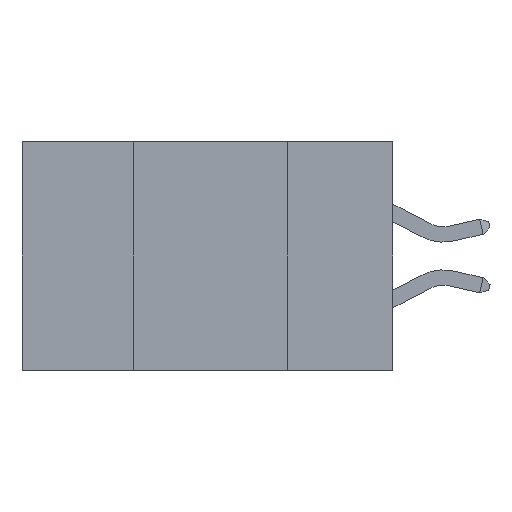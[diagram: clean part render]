
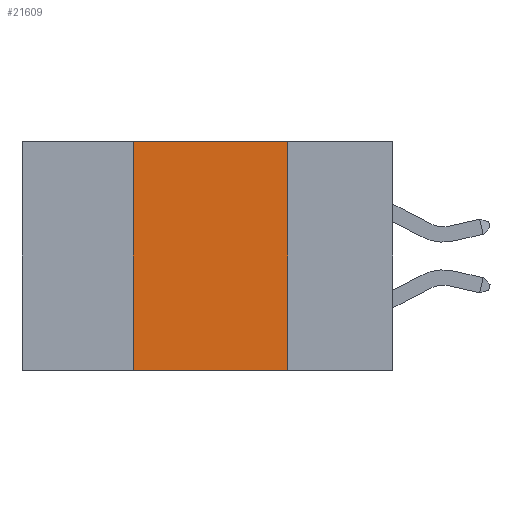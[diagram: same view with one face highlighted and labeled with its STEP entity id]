
A CAD part, left-side view. The second image highlights one B-rep face of the part: STEP entity #21609.
In plain terms, the highlighted planar face has unit normal (-1, 0, 0).
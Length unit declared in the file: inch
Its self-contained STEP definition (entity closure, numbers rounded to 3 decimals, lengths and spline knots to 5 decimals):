
#3584 = DIRECTION ( 'NONE',  ( 1., 0., 0. ) ) ;
#4067 = EDGE_CURVE ( 'NONE', #6951, #6620, #8706, .T. ) ;
#4097 = EDGE_CURVE ( 'NONE', #8169, #19442, #12816, .T. ) ;
#4108 = EDGE_CURVE ( 'NONE', #8169, #6620, #7633, .T. ) ;
#4156 = CARTESIAN_POINT ( 'NONE',  ( 0., 0.42, 0. ) ) ;
#4531 = ORIENTED_EDGE ( 'NONE', *, *, #6141, .F. ) ;
#6141 = EDGE_CURVE ( 'NONE', #19442, #6951, #19881, .T. ) ;
#6620 = VERTEX_POINT ( 'NONE', #16579 ) ;
#6636 = VECTOR ( 'NONE', #17814, 39.37008 ) ;
#6951 = VERTEX_POINT ( 'NONE', #10615 ) ;
#7633 = LINE ( 'NONE', #17028, #16350 ) ;
#8169 = VERTEX_POINT ( 'NONE', #10560 ) ;
#8706 = LINE ( 'NONE', #11692, #17400 ) ;
#9152 = FACE_OUTER_BOUND ( 'NONE', #15309, .T. ) ;
#9955 = DIRECTION ( 'NONE',  ( 0., 0., -1. ) ) ;
#10028 = DIRECTION ( 'NONE',  ( 0., 0., 1. ) ) ;
#10409 = ORIENTED_EDGE ( 'NONE', *, *, #4067, .F. ) ;
#10560 = CARTESIAN_POINT ( 'NONE',  ( 0., 0.42, -0.37 ) ) ;
#10615 = CARTESIAN_POINT ( 'NONE',  ( 0., 0.17, 0. ) ) ;
#11692 = CARTESIAN_POINT ( 'NONE',  ( 0., 0.17, 0. ) ) ;
#12816 = LINE ( 'NONE', #20303, #21325 ) ;
#14296 = PLANE ( 'NONE',  #18950 ) ;
#15309 = EDGE_LOOP ( 'NONE', ( #10409, #4531, #19858, #20445 ) ) ;
#15974 = DIRECTION ( 'NONE',  ( 0., 0., -1. ) ) ;
#16128 = CARTESIAN_POINT ( 'NONE',  ( 0., 0.6, 0. ) ) ;
#16350 = VECTOR ( 'NONE', #18700, 39.37008 ) ;
#16579 = CARTESIAN_POINT ( 'NONE',  ( 0., 0.17, -0.37 ) ) ;
#17028 = CARTESIAN_POINT ( 'NONE',  ( 0., 0.6, -0.37 ) ) ;
#17400 = VECTOR ( 'NONE', #9955, 39.37008 ) ;
#17814 = DIRECTION ( 'NONE',  ( 0., -1., 0. ) ) ;
#18700 = DIRECTION ( 'NONE',  ( 0., -1., 0. ) ) ;
#18950 = AXIS2_PLACEMENT_3D ( 'NONE', #20950, #3584, #15974 ) ;
#19442 = VERTEX_POINT ( 'NONE', #4156 ) ;
#19858 = ORIENTED_EDGE ( 'NONE', *, *, #4097, .F. ) ;
#19881 = LINE ( 'NONE', #16128, #6636 ) ;
#20303 = CARTESIAN_POINT ( 'NONE',  ( 0., 0.42, 0. ) ) ;
#20445 = ORIENTED_EDGE ( 'NONE', *, *, #4108, .T. ) ;
#20950 = CARTESIAN_POINT ( 'NONE',  ( 0., 0.6, 0. ) ) ;
#21325 = VECTOR ( 'NONE', #10028, 39.37008 ) ;
#21609 = ADVANCED_FACE ( 'NONE', ( #9152 ), #14296, .F. ) ;
